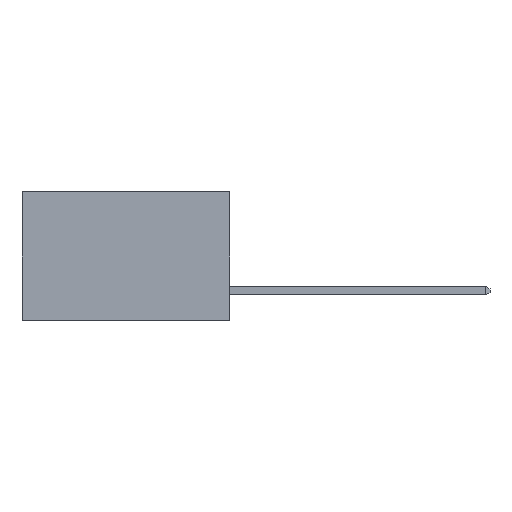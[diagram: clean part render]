
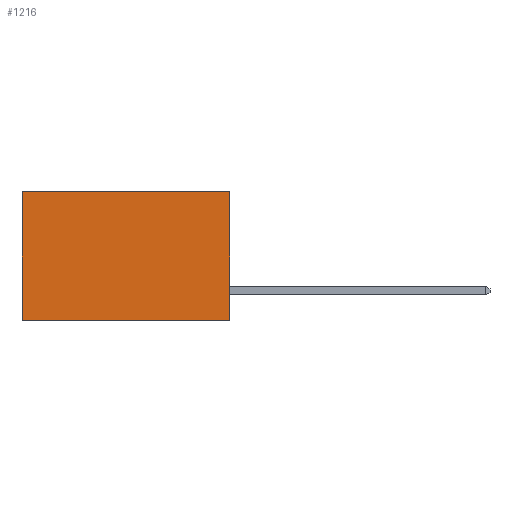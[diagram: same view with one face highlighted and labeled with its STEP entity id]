
A CAD part, left-side view. The second image highlights one B-rep face of the part: STEP entity #1216.
In plain terms, the highlighted planar face has unit normal (-1, 0, 0).
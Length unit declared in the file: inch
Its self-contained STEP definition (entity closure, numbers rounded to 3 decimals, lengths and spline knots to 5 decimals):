
#46 = VERTEX_POINT ( 'NONE', #4924 ) ;
#351 = LINE ( 'NONE', #9044, #9009 ) ;
#796 = EDGE_LOOP ( 'NONE', ( #1915, #1309, #9258, #1840 ) ) ;
#895 = FACE_OUTER_BOUND ( 'NONE', #796, .T. ) ;
#1216 = ADVANCED_FACE ( 'NONE', ( #895 ), #6218, .F. ) ;
#1309 = ORIENTED_EDGE ( 'NONE', *, *, #3734, .F. ) ;
#1536 = CARTESIAN_POINT ( 'NONE',  ( 0.2615, 0.6, -0.37 ) ) ;
#1742 = VECTOR ( 'NONE', #2651, 39.37008 ) ;
#1840 = ORIENTED_EDGE ( 'NONE', *, *, #2859, .T. ) ;
#1915 = ORIENTED_EDGE ( 'NONE', *, *, #4673, .T. ) ;
#2188 = VERTEX_POINT ( 'NONE', #1536 ) ;
#2485 = VERTEX_POINT ( 'NONE', #6786 ) ;
#2579 = LINE ( 'NONE', #5859, #4869 ) ;
#2651 = DIRECTION ( 'NONE',  ( 0., 0., -1. ) ) ;
#2679 = CARTESIAN_POINT ( 'NONE',  ( 0.2615, 0.6, -0.37 ) ) ;
#2859 = EDGE_CURVE ( 'NONE', #3066, #46, #2579, .T. ) ;
#2893 = DIRECTION ( 'NONE',  ( 0., 1., 0. ) ) ;
#3066 = VERTEX_POINT ( 'NONE', #9859 ) ;
#3117 = VECTOR ( 'NONE', #10243, 39.37008 ) ;
#3734 = EDGE_CURVE ( 'NONE', #2485, #2188, #5379, .T. ) ;
#4185 = DIRECTION ( 'NONE',  ( 1., 0., 0. ) ) ;
#4673 = EDGE_CURVE ( 'NONE', #46, #2188, #7979, .T. ) ;
#4869 = VECTOR ( 'NONE', #2893, 39.37008 ) ;
#4924 = CARTESIAN_POINT ( 'NONE',  ( 0.2615, 0.6, 0. ) ) ;
#5228 = AXIS2_PLACEMENT_3D ( 'NONE', #6526, #4185, #7913 ) ;
#5379 = LINE ( 'NONE', #10623, #3117 ) ;
#5496 = EDGE_CURVE ( 'NONE', #3066, #2485, #351, .T. ) ;
#5859 = CARTESIAN_POINT ( 'NONE',  ( 0.2615, 0., 0. ) ) ;
#6218 = PLANE ( 'NONE',  #5228 ) ;
#6526 = CARTESIAN_POINT ( 'NONE',  ( 0.2615, 0., -0.37 ) ) ;
#6786 = CARTESIAN_POINT ( 'NONE',  ( 0.2615, 0., -0.37 ) ) ;
#7913 = DIRECTION ( 'NONE',  ( 0., 0., -1. ) ) ;
#7979 = LINE ( 'NONE', #2679, #1742 ) ;
#8844 = DIRECTION ( 'NONE',  ( 0., 0., -1. ) ) ;
#9009 = VECTOR ( 'NONE', #8844, 39.37008 ) ;
#9044 = CARTESIAN_POINT ( 'NONE',  ( 0.2615, 0., -0.37 ) ) ;
#9258 = ORIENTED_EDGE ( 'NONE', *, *, #5496, .F. ) ;
#9859 = CARTESIAN_POINT ( 'NONE',  ( 0.2615, 0., 0. ) ) ;
#10243 = DIRECTION ( 'NONE',  ( 0., 1., 0. ) ) ;
#10623 = CARTESIAN_POINT ( 'NONE',  ( 0.2615, 0., -0.37 ) ) ;
